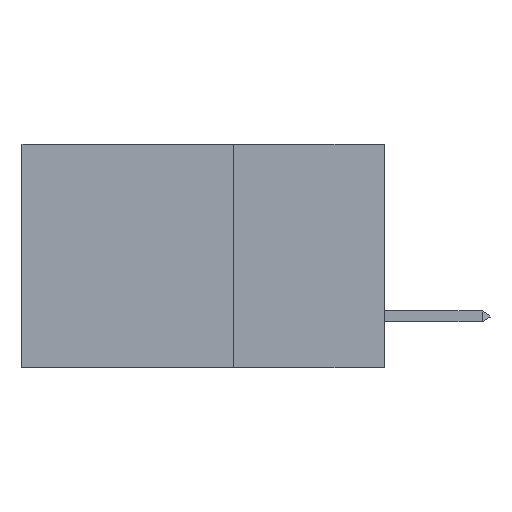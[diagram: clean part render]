
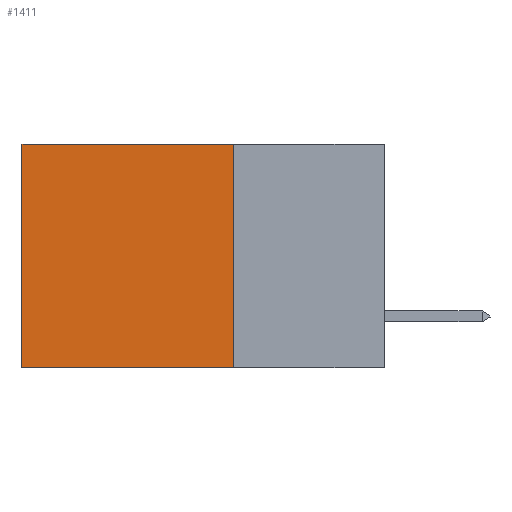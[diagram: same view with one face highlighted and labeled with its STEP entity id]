
A CAD part, left-side view. The second image highlights one B-rep face of the part: STEP entity #1411.
In plain terms, the highlighted planar face has unit normal (-1, 0, 0).
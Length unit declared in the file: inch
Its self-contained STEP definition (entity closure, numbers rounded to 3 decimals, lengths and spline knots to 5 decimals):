
#1411 = ADVANCED_FACE ( 'NONE', ( #10242 ), #2703, .F. ) ;
#2703 = PLANE ( 'NONE',  #12665 ) ;
#3591 = VERTEX_POINT ( 'NONE', #29365 ) ;
#3764 = LINE ( 'NONE', #17997, #30719 ) ;
#6550 = CARTESIAN_POINT ( 'NONE',  ( 0.2875, 0.25, 0. ) ) ;
#6582 = DIRECTION ( 'NONE',  ( 0., 1., 0. ) ) ;
#7660 = VERTEX_POINT ( 'NONE', #19228 ) ;
#8030 = CARTESIAN_POINT ( 'NONE',  ( 0.2875, 0.25, 0. ) ) ;
#10242 = FACE_OUTER_BOUND ( 'NONE', #13849, .T. ) ;
#10603 = DIRECTION ( 'NONE',  ( 0., 0., -1. ) ) ;
#11866 = DIRECTION ( 'NONE',  ( 0., 1., 0. ) ) ;
#12026 = VERTEX_POINT ( 'NONE', #25098 ) ;
#12142 = LINE ( 'NONE', #29299, #47431 ) ;
#12426 = EDGE_CURVE ( 'NONE', #12026, #3591, #32361, .T. ) ;
#12665 = AXIS2_PLACEMENT_3D ( 'NONE', #6550, #37128, #10603 ) ;
#13849 = EDGE_LOOP ( 'NONE', ( #39654, #24274, #15426, #22062 ) ) ;
#15426 = ORIENTED_EDGE ( 'NONE', *, *, #49478, .F. ) ;
#16100 = EDGE_CURVE ( 'NONE', #7660, #28717, #3764, .T. ) ;
#17652 = VECTOR ( 'NONE', #22427, 39.37008 ) ;
#17997 = CARTESIAN_POINT ( 'NONE',  ( 0.2875, 0.25, -0.37 ) ) ;
#19228 = CARTESIAN_POINT ( 'NONE',  ( 0.2875, 0.25, -0.37 ) ) ;
#22062 = ORIENTED_EDGE ( 'NONE', *, *, #12426, .T. ) ;
#22427 = DIRECTION ( 'NONE',  ( 0., 0., -1. ) ) ;
#24274 = ORIENTED_EDGE ( 'NONE', *, *, #16100, .F. ) ;
#25098 = CARTESIAN_POINT ( 'NONE',  ( 0.2875, 0.25, 0. ) ) ;
#25166 = VECTOR ( 'NONE', #11866, 39.37008 ) ;
#25961 = DIRECTION ( 'NONE',  ( 0., 0., -1. ) ) ;
#28717 = VERTEX_POINT ( 'NONE', #40148 ) ;
#29074 = LINE ( 'NONE', #33940, #17652 ) ;
#29299 = CARTESIAN_POINT ( 'NONE',  ( 0.2875, 0.6, 0. ) ) ;
#29365 = CARTESIAN_POINT ( 'NONE',  ( 0.2875, 0.6, 0. ) ) ;
#30719 = VECTOR ( 'NONE', #6582, 39.37008 ) ;
#32361 = LINE ( 'NONE', #8030, #25166 ) ;
#33309 = EDGE_CURVE ( 'NONE', #3591, #28717, #12142, .T. ) ;
#33940 = CARTESIAN_POINT ( 'NONE',  ( 0.2875, 0.25, 0. ) ) ;
#37128 = DIRECTION ( 'NONE',  ( 1., 0., 0. ) ) ;
#39654 = ORIENTED_EDGE ( 'NONE', *, *, #33309, .T. ) ;
#40148 = CARTESIAN_POINT ( 'NONE',  ( 0.2875, 0.6, -0.37 ) ) ;
#47431 = VECTOR ( 'NONE', #25961, 39.37008 ) ;
#49478 = EDGE_CURVE ( 'NONE', #12026, #7660, #29074, .T. ) ;
